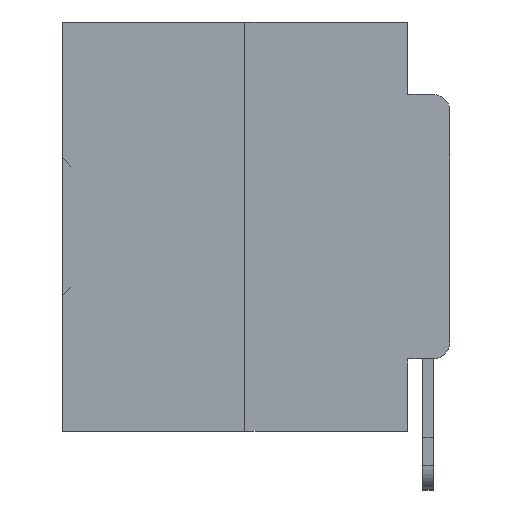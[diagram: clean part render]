
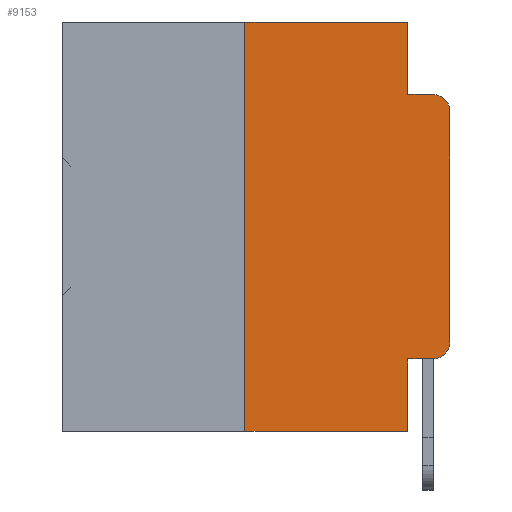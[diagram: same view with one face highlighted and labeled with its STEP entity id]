
A CAD part, left-side view. The second image highlights one B-rep face of the part: STEP entity #9153.
In plain terms, the highlighted planar face has unit normal (-1, 0, 0).
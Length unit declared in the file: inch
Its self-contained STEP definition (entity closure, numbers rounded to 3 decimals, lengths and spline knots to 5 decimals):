
#300 = ORIENTED_EDGE ( 'NONE', *, *, #31380, .T. ) ;
#1240 = ORIENTED_EDGE ( 'NONE', *, *, #21929, .T. ) ;
#1340 = LINE ( 'NONE', #23858, #25136 ) ;
#1518 = VERTEX_POINT ( 'NONE', #25537 ) ;
#1582 = CARTESIAN_POINT ( 'NONE',  ( 0., 0.051, 0. ) ) ;
#1868 = DIRECTION ( 'NONE',  ( 0., 0., -1. ) ) ;
#2170 = ORIENTED_EDGE ( 'NONE', *, *, #37387, .F. ) ;
#2259 = AXIS2_PLACEMENT_3D ( 'NONE', #31172, #19924, #1868 ) ;
#2290 = DIRECTION ( 'NONE',  ( 0., -1., 0. ) ) ;
#2348 = DIRECTION ( 'NONE',  ( 0., 0., -1. ) ) ;
#2754 = VERTEX_POINT ( 'NONE', #1582 ) ;
#3178 = VECTOR ( 'NONE', #8155, 39.37008 ) ;
#3675 = VERTEX_POINT ( 'NONE', #16924 ) ;
#4234 = CARTESIAN_POINT ( 'NONE',  ( 0., 0.02, -0.0885 ) ) ;
#4649 = EDGE_CURVE ( 'NONE', #29385, #27387, #8961, .T. ) ;
#5364 = ORIENTED_EDGE ( 'NONE', *, *, #33853, .F. ) ;
#5469 = ORIENTED_EDGE ( 'NONE', *, *, #20589, .F. ) ;
#5492 = LINE ( 'NONE', #33256, #13598 ) ;
#6186 = CARTESIAN_POINT ( 'NONE',  ( 0., 0., -0.3915 ) ) ;
#6639 = LINE ( 'NONE', #20308, #36308 ) ;
#6755 = CARTESIAN_POINT ( 'NONE',  ( 0., 0.473, 0. ) ) ;
#7163 = FACE_OUTER_BOUND ( 'NONE', #31674, .T. ) ;
#7351 = ORIENTED_EDGE ( 'NONE', *, *, #26442, .F. ) ;
#7623 = DIRECTION ( 'NONE',  ( 0., 0., 1. ) ) ;
#8155 = DIRECTION ( 'NONE',  ( 0., -1., 0. ) ) ;
#8286 = ORIENTED_EDGE ( 'NONE', *, *, #14914, .T. ) ;
#8961 = CIRCLE ( 'NONE', #12836, 0.02 ) ;
#9031 = ORIENTED_EDGE ( 'NONE', *, *, #20699, .F. ) ;
#9153 = ADVANCED_FACE ( 'NONE', ( #7163 ), #36550, .F. ) ;
#9426 = CARTESIAN_POINT ( 'NONE',  ( 0., 0.051, -0.0885 ) ) ;
#9851 = DIRECTION ( 'NONE',  ( 0., -1., 0. ) ) ;
#10293 = LINE ( 'NONE', #6755, #16429 ) ;
#10306 = ORIENTED_EDGE ( 'NONE', *, *, #18772, .T. ) ;
#10385 = ORIENTED_EDGE ( 'NONE', *, *, #4649, .T. ) ;
#10502 = CARTESIAN_POINT ( 'NONE',  ( 0., 0.051, -0.0885 ) ) ;
#11309 = LINE ( 'NONE', #25819, #3178 ) ;
#12698 = VERTEX_POINT ( 'NONE', #10502 ) ;
#12836 = AXIS2_PLACEMENT_3D ( 'NONE', #29879, #15665, #29766 ) ;
#13598 = VECTOR ( 'NONE', #30365, 39.37008 ) ;
#14044 = CARTESIAN_POINT ( 'NONE',  ( 0., 0.051, -0.4115 ) ) ;
#14914 = EDGE_CURVE ( 'NONE', #1518, #3675, #6639, .T. ) ;
#15497 = LINE ( 'NONE', #24463, #36958 ) ;
#15665 = DIRECTION ( 'NONE',  ( -1., 0., 0. ) ) ;
#16429 = VECTOR ( 'NONE', #9851, 39.37008 ) ;
#16518 = CARTESIAN_POINT ( 'NONE',  ( 0., 0.25, 0. ) ) ;
#16924 = CARTESIAN_POINT ( 'NONE',  ( 0., 0.051, -0.5 ) ) ;
#17519 = AXIS2_PLACEMENT_3D ( 'NONE', #36949, #20363, #2348 ) ;
#18338 = LINE ( 'NONE', #9426, #34167 ) ;
#18772 = EDGE_CURVE ( 'NONE', #27677, #29385, #11309, .T. ) ;
#19036 = CIRCLE ( 'NONE', #17519, 0.02 ) ;
#19887 = VERTEX_POINT ( 'NONE', #27112 ) ;
#19924 = DIRECTION ( 'NONE',  ( 1., 0., 0. ) ) ;
#20308 = CARTESIAN_POINT ( 'NONE',  ( 0., 0.473, -0.5 ) ) ;
#20363 = DIRECTION ( 'NONE',  ( -1., 0., 0. ) ) ;
#20589 = EDGE_CURVE ( 'NONE', #19887, #2754, #10293, .T. ) ;
#20699 = EDGE_CURVE ( 'NONE', #27677, #3675, #5492, .T. ) ;
#20741 = VERTEX_POINT ( 'NONE', #4234 ) ;
#21357 = DIRECTION ( 'NONE',  ( 0., -1., 0. ) ) ;
#21569 = DIRECTION ( 'NONE',  ( 0., 0., -1. ) ) ;
#21929 = EDGE_CURVE ( 'NONE', #36997, #20741, #19036, .T. ) ;
#23858 = CARTESIAN_POINT ( 'NONE',  ( 0., 0., 0. ) ) ;
#24463 = CARTESIAN_POINT ( 'NONE',  ( 0., 0.051, 0. ) ) ;
#25136 = VECTOR ( 'NONE', #32166, 39.37008 ) ;
#25523 = CARTESIAN_POINT ( 'NONE',  ( 0., 0., -0.1085 ) ) ;
#25537 = CARTESIAN_POINT ( 'NONE',  ( 0., 0.25, -0.5 ) ) ;
#25819 = CARTESIAN_POINT ( 'NONE',  ( 0., 0.051, -0.4115 ) ) ;
#26442 = EDGE_CURVE ( 'NONE', #1518, #19887, #36666, .T. ) ;
#27112 = CARTESIAN_POINT ( 'NONE',  ( 0., 0.25, 0. ) ) ;
#27387 = VERTEX_POINT ( 'NONE', #6186 ) ;
#27677 = VERTEX_POINT ( 'NONE', #14044 ) ;
#29385 = VERTEX_POINT ( 'NONE', #36583 ) ;
#29766 = DIRECTION ( 'NONE',  ( 0., 0., -1. ) ) ;
#29879 = CARTESIAN_POINT ( 'NONE',  ( 0., 0.02, -0.3915 ) ) ;
#30365 = DIRECTION ( 'NONE',  ( 0., 0., -1. ) ) ;
#31172 = CARTESIAN_POINT ( 'NONE',  ( 0., 0.473, 0. ) ) ;
#31380 = EDGE_CURVE ( 'NONE', #27387, #36997, #1340, .T. ) ;
#31674 = EDGE_LOOP ( 'NONE', ( #300, #1240, #2170, #5364, #5469, #7351, #8286, #9031, #10306, #10385 ) ) ;
#32166 = DIRECTION ( 'NONE',  ( 0., 0., 1. ) ) ;
#33256 = CARTESIAN_POINT ( 'NONE',  ( 0., 0.051, 0. ) ) ;
#33853 = EDGE_CURVE ( 'NONE', #2754, #12698, #15497, .T. ) ;
#34167 = VECTOR ( 'NONE', #21357, 39.37008 ) ;
#35814 = VECTOR ( 'NONE', #7623, 39.37008 ) ;
#36308 = VECTOR ( 'NONE', #2290, 39.37008 ) ;
#36550 = PLANE ( 'NONE',  #2259 ) ;
#36583 = CARTESIAN_POINT ( 'NONE',  ( 0., 0.02, -0.4115 ) ) ;
#36666 = LINE ( 'NONE', #16518, #35814 ) ;
#36949 = CARTESIAN_POINT ( 'NONE',  ( 0., 0.02, -0.1085 ) ) ;
#36958 = VECTOR ( 'NONE', #21569, 39.37008 ) ;
#36997 = VERTEX_POINT ( 'NONE', #25523 ) ;
#37387 = EDGE_CURVE ( 'NONE', #12698, #20741, #18338, .T. ) ;
